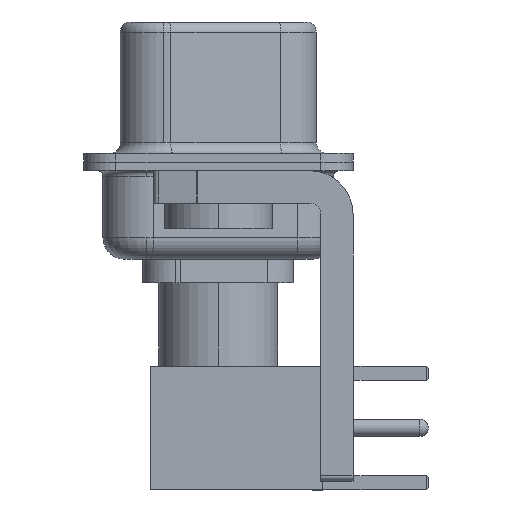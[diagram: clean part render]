
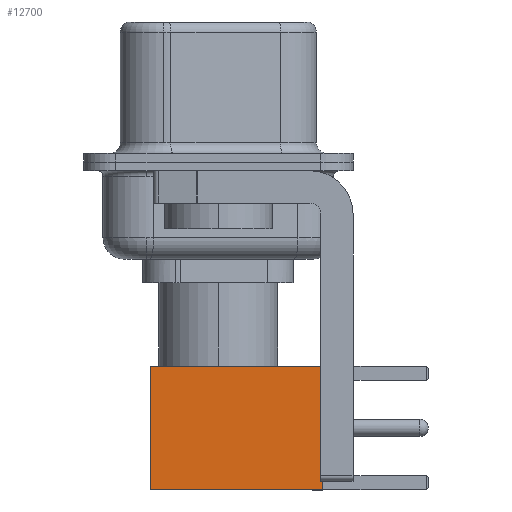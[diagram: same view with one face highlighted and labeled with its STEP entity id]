
A CAD part, left-side view. The second image highlights one B-rep face of the part: STEP entity #12700.
In plain terms, the highlighted face is planar.
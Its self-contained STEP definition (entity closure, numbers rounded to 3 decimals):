
#603 = DIRECTION ( 'NONE',  ( 0., 0., 1. ) ) ;
#2331 = VERTEX_POINT ( 'NONE', #3124 ) ;
#2823 = CARTESIAN_POINT ( 'NONE',  ( 0., 2.875, 0. ) ) ;
#3112 = LINE ( 'NONE', #11837, #3556 ) ;
#3124 = CARTESIAN_POINT ( 'NONE',  ( 2.875, 2.875, 0. ) ) ;
#3544 = VECTOR ( 'NONE', #17036, 1000. ) ;
#3556 = VECTOR ( 'NONE', #10373, 1000. ) ;
#3649 = ORIENTED_EDGE ( 'NONE', *, *, #11513, .T. ) ;
#5857 = EDGE_LOOP ( 'NONE', ( #18359, #3649, #8916, #12859 ) ) ;
#5901 = CARTESIAN_POINT ( 'NONE',  ( -2.875, 2.875, 0. ) ) ;
#7179 = LINE ( 'NONE', #8306, #15794 ) ;
#7590 = PLANE ( 'NONE',  #13124 ) ;
#7777 = CARTESIAN_POINT ( 'NONE',  ( -2.875, 2.875, 8. ) ) ;
#8306 = CARTESIAN_POINT ( 'NONE',  ( -2.875, 2.875, 0. ) ) ;
#8876 = EDGE_CURVE ( 'NONE', #18004, #17834, #14035, .T. ) ;
#8916 = ORIENTED_EDGE ( 'NONE', *, *, #9961, .F. ) ;
#9961 = EDGE_CURVE ( 'NONE', #17834, #11149, #7179, .T. ) ;
#10373 = DIRECTION ( 'NONE',  ( 0., 0., -1. ) ) ;
#11149 = VERTEX_POINT ( 'NONE', #5901 ) ;
#11210 = EDGE_CURVE ( 'NONE', #18004, #2331, #3112, .T. ) ;
#11513 = EDGE_CURVE ( 'NONE', #2331, #11149, #14103, .T. ) ;
#11837 = CARTESIAN_POINT ( 'NONE',  ( 2.875, 2.875, 0. ) ) ;
#12700 = ADVANCED_FACE ( 'NONE', ( #13352 ), #7590, .T. ) ;
#12859 = ORIENTED_EDGE ( 'NONE', *, *, #8876, .F. ) ;
#13124 = AXIS2_PLACEMENT_3D ( 'NONE', #13446, #13267, #603 ) ;
#13267 = DIRECTION ( 'NONE',  ( 0., 1., 0. ) ) ;
#13352 = FACE_OUTER_BOUND ( 'NONE', #5857, .T. ) ;
#13446 = CARTESIAN_POINT ( 'NONE',  ( 2.875, 2.875, 0. ) ) ;
#13990 = DIRECTION ( 'NONE',  ( 0., 0., -1. ) ) ;
#14035 = LINE ( 'NONE', #18426, #3544 ) ;
#14103 = LINE ( 'NONE', #2823, #16083 ) ;
#15250 = CARTESIAN_POINT ( 'NONE',  ( 2.875, 2.875, 8. ) ) ;
#15794 = VECTOR ( 'NONE', #13990, 1000. ) ;
#16083 = VECTOR ( 'NONE', #18203, 1000. ) ;
#17036 = DIRECTION ( 'NONE',  ( -1., 0., 0. ) ) ;
#17834 = VERTEX_POINT ( 'NONE', #7777 ) ;
#18004 = VERTEX_POINT ( 'NONE', #15250 ) ;
#18203 = DIRECTION ( 'NONE',  ( -1., 0., 0. ) ) ;
#18359 = ORIENTED_EDGE ( 'NONE', *, *, #11210, .T. ) ;
#18426 = CARTESIAN_POINT ( 'NONE',  ( 0., 2.875, 8. ) ) ;
